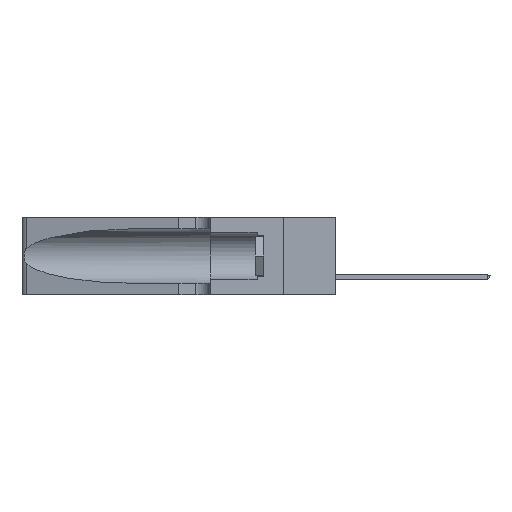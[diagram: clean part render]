
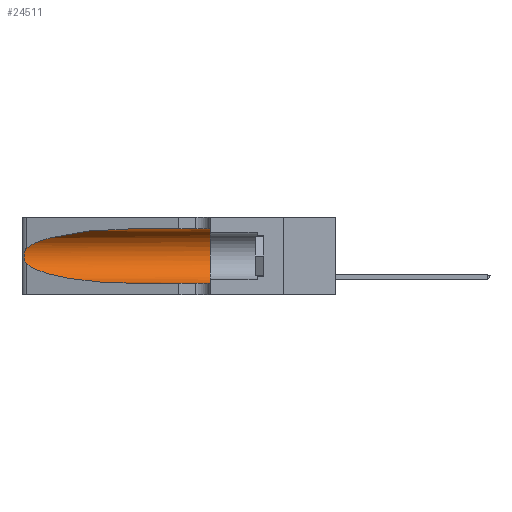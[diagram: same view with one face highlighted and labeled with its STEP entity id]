
A CAD part, left-side view. The second image highlights one B-rep face of the part: STEP entity #24511.
In plain terms, the highlighted cylindrical face has radius 3.308 mm (diameter 6.617 mm), a partial arc.
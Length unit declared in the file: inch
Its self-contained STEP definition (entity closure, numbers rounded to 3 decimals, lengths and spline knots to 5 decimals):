
#944 = EDGE_CURVE ( 'NONE', #5513, #13791, #27191, .T. ) ;
#1423 = CARTESIAN_POINT ( 'NONE',  ( 0.18966, 0.96281, 0.31525 ) ) ;
#1600 =( BOUNDED_CURVE ( )  B_SPLINE_CURVE ( 3, ( #29630, #1423, #10080, #35138 ),
 .UNSPECIFIED., .F., .F. ) 
 B_SPLINE_CURVE_WITH_KNOTS ( ( 4, 4 ),
 ( 1.5708, 2.84003 ),
 .UNSPECIFIED. ) 
 CURVE ( )  GEOMETRIC_REPRESENTATION_ITEM ( )  RATIONAL_B_SPLINE_CURVE ( ( 1., 0.87, 0.87, 1. ) ) 
 REPRESENTATION_ITEM ( '' )  );
#2215 = VECTOR ( 'NONE', #30963, 39.37008 ) ;
#2804 = CARTESIAN_POINT ( 'NONE',  ( 0.26017, 1.23833, 0.17102 ) ) ;
#3236 = CARTESIAN_POINT ( 'NONE',  ( 0.25487, 1.22718, 0.22369 ) ) ;
#3442 = VECTOR ( 'NONE', #35633, 39.37008 ) ;
#3507 = CARTESIAN_POINT ( 'NONE',  ( 0.25555, 1.22994, 0.2215 ) ) ;
#3827 = B_SPLINE_CURVE_WITH_KNOTS ( 'NONE', 3,
 ( #8931, #3507, #19943, #21672, #21287, #25273, #28768, #23123, #2804, #19463, #22223, #16508, #13512, #8305 ),
 .UNSPECIFIED., .F., .F.,
 ( 4, 2, 2, 2, 2, 2, 4 ),
 ( 0., 0.00027, 0.00053, 0.00107, 0.0016, 0.00187, 0.00214 ),
 .UNSPECIFIED. ) ;
#4343 = CARTESIAN_POINT ( 'NONE',  ( 0.1305, 0.72297, 0.05475 ) ) ;
#5201 = EDGE_CURVE ( 'NONE', #21642, #13791, #10047, .T. ) ;
#5513 = VERTEX_POINT ( 'NONE', #8186 ) ;
#7092 = DIRECTION ( 'NONE',  ( 0., -1., 0. ) ) ;
#7772 = DIRECTION ( 'NONE',  ( 0., 1., 0. ) ) ;
#7916 = FACE_OUTER_BOUND ( 'NONE', #35215, .T. ) ;
#7995 = CARTESIAN_POINT ( 'NONE',  ( 0.1305, 0.72297, 0.05475 ) ) ;
#8144 = VERTEX_POINT ( 'NONE', #20483 ) ;
#8186 = CARTESIAN_POINT ( 'NONE',  ( 0.1305, 0.35, 0.31525 ) ) ;
#8305 = CARTESIAN_POINT ( 'NONE',  ( 0.25487, 1.22718, 0.14631 ) ) ;
#8320 = CYLINDRICAL_SURFACE ( 'NONE', #11474, 0.13025 ) ;
#8931 = CARTESIAN_POINT ( 'NONE',  ( 0.25487, 1.22718, 0.22369 ) ) ;
#9130 = ORIENTED_EDGE ( 'NONE', *, *, #15088, .T. ) ;
#9527 = LINE ( 'NONE', #32855, #3442 ) ;
#10047 = LINE ( 'NONE', #29561, #2215 ) ;
#10080 = CARTESIAN_POINT ( 'NONE',  ( 0.2373, 1.15595, 0.28018 ) ) ;
#10740 = CARTESIAN_POINT ( 'NONE',  ( 0.1305, 0.35, 0.05475 ) ) ;
#11009 = EDGE_CURVE ( 'NONE', #20908, #5513, #9527, .T. ) ;
#11474 = AXIS2_PLACEMENT_3D ( 'NONE', #31882, #7092, #20670 ) ;
#13512 = CARTESIAN_POINT ( 'NONE',  ( 0.25555, 1.22993, 0.14849 ) ) ;
#13548 = CARTESIAN_POINT ( 'NONE',  ( 0.25487, 1.22718, 0.14631 ) ) ;
#13791 = VERTEX_POINT ( 'NONE', #10740 ) ;
#13877 = ORIENTED_EDGE ( 'NONE', *, *, #5201, .T. ) ;
#14203 = VERTEX_POINT ( 'NONE', #3236 ) ;
#15088 = EDGE_CURVE ( 'NONE', #14203, #8144, #3827, .T. ) ;
#16508 = CARTESIAN_POINT ( 'NONE',  ( 0.25639, 1.23186, 0.15144 ) ) ;
#17020 = ORIENTED_EDGE ( 'NONE', *, *, #944, .F. ) ;
#19463 = CARTESIAN_POINT ( 'NONE',  ( 0.25856, 1.23593, 0.16098 ) ) ;
#19943 = CARTESIAN_POINT ( 'NONE',  ( 0.25639, 1.23184, 0.21858 ) ) ;
#20483 = CARTESIAN_POINT ( 'NONE',  ( 0.25487, 1.22718, 0.14631 ) ) ;
#20670 = DIRECTION ( 'NONE',  ( 0., 0., -1. ) ) ;
#20908 = VERTEX_POINT ( 'NONE', #23168 ) ;
#21121 = AXIS2_PLACEMENT_3D ( 'NONE', #30212, #7772, #30436 ) ;
#21287 = CARTESIAN_POINT ( 'NONE',  ( 0.25854, 1.2359, 0.20912 ) ) ;
#21642 = VERTEX_POINT ( 'NONE', #4343 ) ;
#21672 = CARTESIAN_POINT ( 'NONE',  ( 0.25787, 1.23484, 0.2124 ) ) ;
#22223 = CARTESIAN_POINT ( 'NONE',  ( 0.25789, 1.23486, 0.15765 ) ) ;
#23123 = CARTESIAN_POINT ( 'NONE',  ( 0.26075, 1.23896, 0.178 ) ) ;
#23168 = CARTESIAN_POINT ( 'NONE',  ( 0.1305, 0.72297, 0.31525 ) ) ;
#23877 = ORIENTED_EDGE ( 'NONE', *, *, #11009, .F. ) ;
#24379 = ORIENTED_EDGE ( 'NONE', *, *, #27995, .T. ) ;
#24511 = ADVANCED_FACE ( 'NONE', ( #7916 ), #8320, .F. ) ;
#25273 = CARTESIAN_POINT ( 'NONE',  ( 0.26018, 1.23835, 0.19895 ) ) ;
#27191 = CIRCLE ( 'NONE', #21121, 0.13025 ) ;
#27995 = EDGE_CURVE ( 'NONE', #8144, #21642, #29195, .T. ) ;
#28732 = EDGE_CURVE ( 'NONE', #20908, #14203, #1600, .T. ) ;
#28768 = CARTESIAN_POINT ( 'NONE',  ( 0.26075, 1.23896, 0.19203 ) ) ;
#29195 =( BOUNDED_CURVE ( )  B_SPLINE_CURVE ( 3, ( #13548, #35719, #32681, #7995 ),
 .UNSPECIFIED., .F., .F. ) 
 B_SPLINE_CURVE_WITH_KNOTS ( ( 4, 4 ),
 ( 3.44316, 4.71239 ),
 .UNSPECIFIED. ) 
 CURVE ( )  GEOMETRIC_REPRESENTATION_ITEM ( )  RATIONAL_B_SPLINE_CURVE ( ( 1., 0.87, 0.87, 1. ) ) 
 REPRESENTATION_ITEM ( '' )  );
#29561 = CARTESIAN_POINT ( 'NONE',  ( 0.1305, 1.61858, 0.05475 ) ) ;
#29630 = CARTESIAN_POINT ( 'NONE',  ( 0.1305, 0.72297, 0.31525 ) ) ;
#30193 = ORIENTED_EDGE ( 'NONE', *, *, #28732, .T. ) ;
#30212 = CARTESIAN_POINT ( 'NONE',  ( 0.1305, 0.35, 0.185 ) ) ;
#30436 = DIRECTION ( 'NONE',  ( 0., 0., 1. ) ) ;
#30963 = DIRECTION ( 'NONE',  ( 0., -1., 0. ) ) ;
#31882 = CARTESIAN_POINT ( 'NONE',  ( 0.1305, 1.61858, 0.185 ) ) ;
#32681 = CARTESIAN_POINT ( 'NONE',  ( 0.18966, 0.96281, 0.05475 ) ) ;
#32855 = CARTESIAN_POINT ( 'NONE',  ( 0.1305, 1.61858, 0.31525 ) ) ;
#35138 = CARTESIAN_POINT ( 'NONE',  ( 0.25487, 1.22718, 0.22369 ) ) ;
#35215 = EDGE_LOOP ( 'NONE', ( #30193, #9130, #24379, #13877, #17020, #23877 ) ) ;
#35633 = DIRECTION ( 'NONE',  ( 0., -1., 0. ) ) ;
#35719 = CARTESIAN_POINT ( 'NONE',  ( 0.2373, 1.15595, 0.08982 ) ) ;
